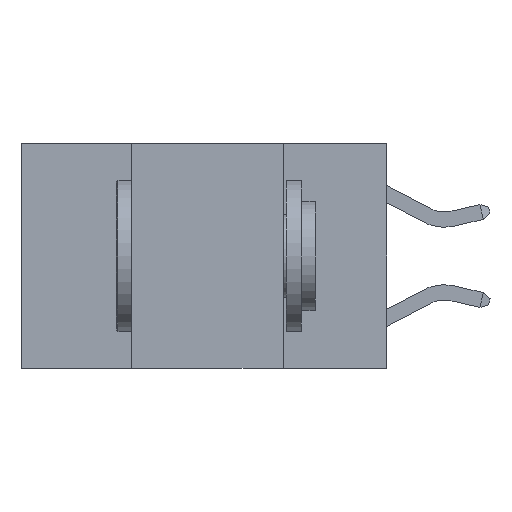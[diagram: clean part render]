
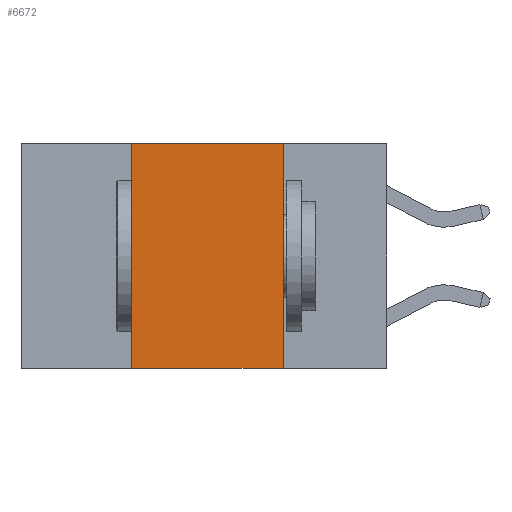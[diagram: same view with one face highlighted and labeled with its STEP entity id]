
A CAD part, left-side view. The second image highlights one B-rep face of the part: STEP entity #6672.
In plain terms, the highlighted planar face has unit normal (-1, 0, 0).
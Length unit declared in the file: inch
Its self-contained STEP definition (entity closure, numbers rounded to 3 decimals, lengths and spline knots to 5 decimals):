
#158 = CARTESIAN_POINT ( 'NONE',  ( 0., 0.17, -0.37 ) ) ;
#587 = DIRECTION ( 'NONE',  ( 0., 0., -1. ) ) ;
#607 = VERTEX_POINT ( 'NONE', #158 ) ;
#717 = VERTEX_POINT ( 'NONE', #11974 ) ;
#1226 = CARTESIAN_POINT ( 'NONE',  ( 0., 0.17, 0. ) ) ;
#1363 = CARTESIAN_POINT ( 'NONE',  ( 0., 0.42, 0. ) ) ;
#1535 = PLANE ( 'NONE',  #9138 ) ;
#1992 = VECTOR ( 'NONE', #10959, 39.37008 ) ;
#3107 = EDGE_CURVE ( 'NONE', #8445, #9045, #10454, .T. ) ;
#3302 = EDGE_LOOP ( 'NONE', ( #3674, #8668, #6453, #4549 ) ) ;
#3674 = ORIENTED_EDGE ( 'NONE', *, *, #5624, .F. ) ;
#4168 = VECTOR ( 'NONE', #12252, 39.37008 ) ;
#4340 = VECTOR ( 'NONE', #7845, 39.37008 ) ;
#4364 = EDGE_CURVE ( 'NONE', #8445, #607, #4520, .T. ) ;
#4411 = CARTESIAN_POINT ( 'NONE',  ( 0., 0.6, 0. ) ) ;
#4520 = LINE ( 'NONE', #9976, #1992 ) ;
#4549 = ORIENTED_EDGE ( 'NONE', *, *, #4364, .T. ) ;
#4579 = CARTESIAN_POINT ( 'NONE',  ( 0., 0.42, 0. ) ) ;
#5624 = EDGE_CURVE ( 'NONE', #717, #607, #11914, .T. ) ;
#6300 = DIRECTION ( 'NONE',  ( 1., 0., 0. ) ) ;
#6381 = LINE ( 'NONE', #8433, #4168 ) ;
#6453 = ORIENTED_EDGE ( 'NONE', *, *, #3107, .F. ) ;
#6672 = ADVANCED_FACE ( 'NONE', ( #10692 ), #1535, .F. ) ;
#6806 = EDGE_CURVE ( 'NONE', #9045, #717, #6381, .T. ) ;
#7328 = VECTOR ( 'NONE', #11845, 39.37008 ) ;
#7845 = DIRECTION ( 'NONE',  ( 0., 0., -1. ) ) ;
#8433 = CARTESIAN_POINT ( 'NONE',  ( 0., 0.6, 0. ) ) ;
#8445 = VERTEX_POINT ( 'NONE', #9834 ) ;
#8668 = ORIENTED_EDGE ( 'NONE', *, *, #6806, .F. ) ;
#9045 = VERTEX_POINT ( 'NONE', #4579 ) ;
#9138 = AXIS2_PLACEMENT_3D ( 'NONE', #4411, #6300, #587 ) ;
#9834 = CARTESIAN_POINT ( 'NONE',  ( 0., 0.42, -0.37 ) ) ;
#9976 = CARTESIAN_POINT ( 'NONE',  ( 0., 0.6, -0.37 ) ) ;
#10454 = LINE ( 'NONE', #1363, #7328 ) ;
#10692 = FACE_OUTER_BOUND ( 'NONE', #3302, .T. ) ;
#10959 = DIRECTION ( 'NONE',  ( 0., -1., 0. ) ) ;
#11845 = DIRECTION ( 'NONE',  ( 0., 0., 1. ) ) ;
#11914 = LINE ( 'NONE', #1226, #4340 ) ;
#11974 = CARTESIAN_POINT ( 'NONE',  ( 0., 0.17, 0. ) ) ;
#12252 = DIRECTION ( 'NONE',  ( 0., -1., 0. ) ) ;
